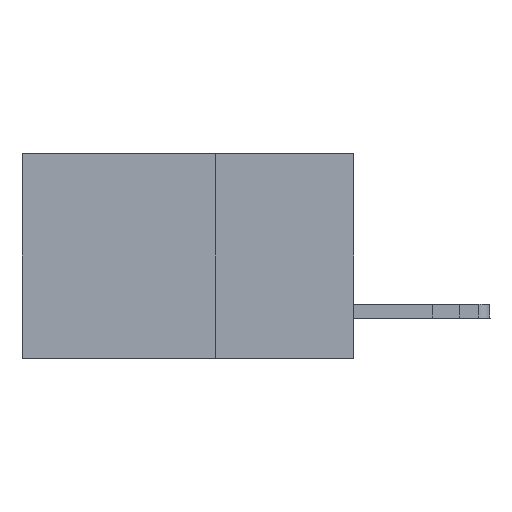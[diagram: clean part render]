
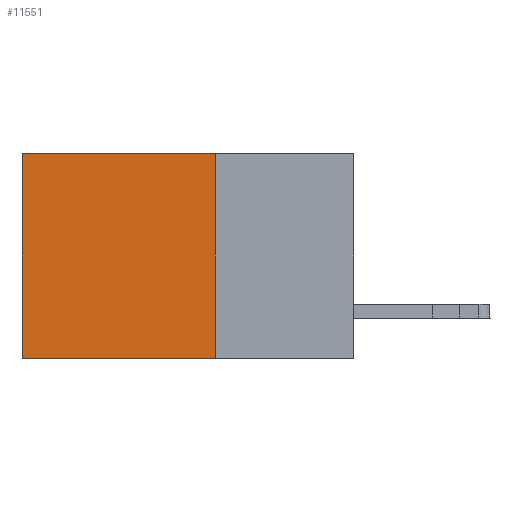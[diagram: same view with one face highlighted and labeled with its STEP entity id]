
A CAD part, left-side view. The second image highlights one B-rep face of the part: STEP entity #11551.
In plain terms, the highlighted planar face has unit normal (-1, 0, 0).
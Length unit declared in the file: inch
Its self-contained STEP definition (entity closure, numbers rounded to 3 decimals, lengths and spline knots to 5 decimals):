
#216 = LINE ( 'NONE', #16219, #10259 ) ;
#988 = CARTESIAN_POINT ( 'NONE',  ( 0.2875, 0.25, -0.37 ) ) ;
#1446 = EDGE_CURVE ( 'NONE', #13508, #2775, #6900, .T. ) ;
#1447 = CARTESIAN_POINT ( 'NONE',  ( 0.2875, 0.25, 0. ) ) ;
#1944 = DIRECTION ( 'NONE',  ( 0., 0., -1. ) ) ;
#2775 = VERTEX_POINT ( 'NONE', #988 ) ;
#2830 = DIRECTION ( 'NONE',  ( 0., 0., -1. ) ) ;
#3415 = EDGE_CURVE ( 'NONE', #13508, #15126, #10968, .T. ) ;
#3732 = CARTESIAN_POINT ( 'NONE',  ( 0.2875, 0.25, 0. ) ) ;
#3927 = VERTEX_POINT ( 'NONE', #14782 ) ;
#5082 = LINE ( 'NONE', #13582, #11018 ) ;
#5134 = EDGE_LOOP ( 'NONE', ( #6290, #6778, #16554, #6554 ) ) ;
#5465 = PLANE ( 'NONE',  #6027 ) ;
#6027 = AXIS2_PLACEMENT_3D ( 'NONE', #15505, #10542, #2830 ) ;
#6290 = ORIENTED_EDGE ( 'NONE', *, *, #15568, .T. ) ;
#6554 = ORIENTED_EDGE ( 'NONE', *, *, #3415, .T. ) ;
#6778 = ORIENTED_EDGE ( 'NONE', *, *, #11914, .F. ) ;
#6900 = LINE ( 'NONE', #1447, #9841 ) ;
#7483 = DIRECTION ( 'NONE',  ( 0., 1., 0. ) ) ;
#8031 = VECTOR ( 'NONE', #13815, 39.37008 ) ;
#9475 = FACE_OUTER_BOUND ( 'NONE', #5134, .T. ) ;
#9841 = VECTOR ( 'NONE', #1944, 39.37008 ) ;
#10259 = VECTOR ( 'NONE', #7483, 39.37008 ) ;
#10542 = DIRECTION ( 'NONE',  ( 1., 0., 0. ) ) ;
#10968 = LINE ( 'NONE', #3732, #8031 ) ;
#11018 = VECTOR ( 'NONE', #16074, 39.37008 ) ;
#11551 = ADVANCED_FACE ( 'NONE', ( #9475 ), #5465, .F. ) ;
#11914 = EDGE_CURVE ( 'NONE', #2775, #3927, #216, .T. ) ;
#12275 = CARTESIAN_POINT ( 'NONE',  ( 0.2875, 0.25, 0. ) ) ;
#13508 = VERTEX_POINT ( 'NONE', #12275 ) ;
#13582 = CARTESIAN_POINT ( 'NONE',  ( 0.2875, 0.6, 0. ) ) ;
#13815 = DIRECTION ( 'NONE',  ( 0., 1., 0. ) ) ;
#14782 = CARTESIAN_POINT ( 'NONE',  ( 0.2875, 0.6, -0.37 ) ) ;
#15126 = VERTEX_POINT ( 'NONE', #16354 ) ;
#15505 = CARTESIAN_POINT ( 'NONE',  ( 0.2875, 0.25, 0. ) ) ;
#15568 = EDGE_CURVE ( 'NONE', #15126, #3927, #5082, .T. ) ;
#16074 = DIRECTION ( 'NONE',  ( 0., 0., -1. ) ) ;
#16219 = CARTESIAN_POINT ( 'NONE',  ( 0.2875, 0.25, -0.37 ) ) ;
#16354 = CARTESIAN_POINT ( 'NONE',  ( 0.2875, 0.6, 0. ) ) ;
#16554 = ORIENTED_EDGE ( 'NONE', *, *, #1446, .F. ) ;
